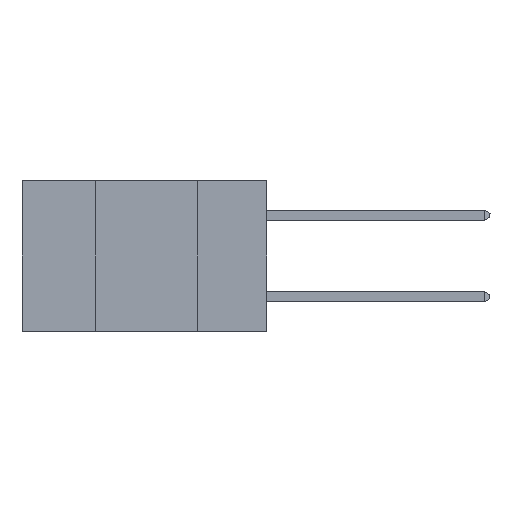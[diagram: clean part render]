
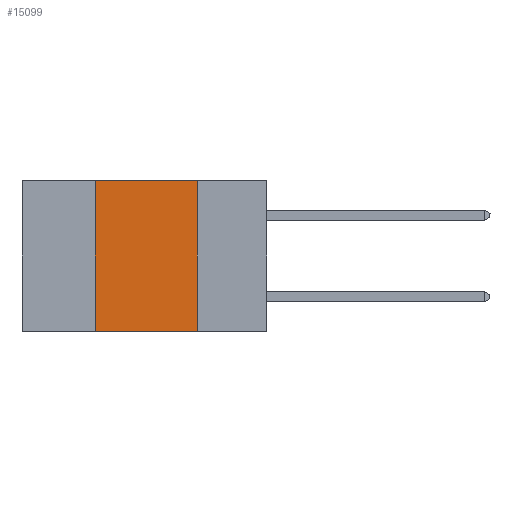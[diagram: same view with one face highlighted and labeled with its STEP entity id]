
A CAD part, left-side view. The second image highlights one B-rep face of the part: STEP entity #15099.
In plain terms, the highlighted planar face has unit normal (-1, 0, 0).
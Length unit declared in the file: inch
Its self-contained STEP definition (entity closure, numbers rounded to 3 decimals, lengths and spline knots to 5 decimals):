
#462 = CARTESIAN_POINT ( 'NONE',  ( 0., 0.42, 0. ) ) ;
#1358 = VECTOR ( 'NONE', #18595, 39.37008 ) ;
#1418 = EDGE_LOOP ( 'NONE', ( #22728, #8072, #20834, #23311 ) ) ;
#2671 = CARTESIAN_POINT ( 'NONE',  ( 0., 0.6, 0. ) ) ;
#7929 = VERTEX_POINT ( 'NONE', #19419 ) ;
#8072 = ORIENTED_EDGE ( 'NONE', *, *, #17607, .F. ) ;
#9355 = CARTESIAN_POINT ( 'NONE',  ( 0., 0.42, -0.37 ) ) ;
#9551 = VERTEX_POINT ( 'NONE', #22635 ) ;
#10447 = LINE ( 'NONE', #24664, #15486 ) ;
#10611 = DIRECTION ( 'NONE',  ( 0., 0., -1. ) ) ;
#10777 = LINE ( 'NONE', #20948, #1358 ) ;
#10842 = DIRECTION ( 'NONE',  ( 0., 0., 1. ) ) ;
#10975 = AXIS2_PLACEMENT_3D ( 'NONE', #2671, #24427, #10611 ) ;
#11197 = VERTEX_POINT ( 'NONE', #462 ) ;
#11290 = CARTESIAN_POINT ( 'NONE',  ( 0., 0.6, -0.37 ) ) ;
#11624 = VECTOR ( 'NONE', #19224, 39.37008 ) ;
#15099 = ADVANCED_FACE ( 'NONE', ( #20758 ), #20510, .F. ) ;
#15486 = VECTOR ( 'NONE', #10842, 39.37008 ) ;
#16877 = EDGE_CURVE ( 'NONE', #20349, #11197, #10447, .T. ) ;
#17493 = CARTESIAN_POINT ( 'NONE',  ( 0., 0.17, 0. ) ) ;
#17607 = EDGE_CURVE ( 'NONE', #11197, #7929, #10777, .T. ) ;
#18595 = DIRECTION ( 'NONE',  ( 0., -1., 0. ) ) ;
#19224 = DIRECTION ( 'NONE',  ( 0., -1., 0. ) ) ;
#19419 = CARTESIAN_POINT ( 'NONE',  ( 0., 0.17, 0. ) ) ;
#19437 = LINE ( 'NONE', #17493, #24631 ) ;
#20349 = VERTEX_POINT ( 'NONE', #9355 ) ;
#20510 = PLANE ( 'NONE',  #10975 ) ;
#20758 = FACE_OUTER_BOUND ( 'NONE', #1418, .T. ) ;
#20834 = ORIENTED_EDGE ( 'NONE', *, *, #16877, .F. ) ;
#20948 = CARTESIAN_POINT ( 'NONE',  ( 0., 0.6, 0. ) ) ;
#21173 = LINE ( 'NONE', #11290, #11624 ) ;
#21337 = EDGE_CURVE ( 'NONE', #7929, #9551, #19437, .T. ) ;
#22635 = CARTESIAN_POINT ( 'NONE',  ( 0., 0.17, -0.37 ) ) ;
#22728 = ORIENTED_EDGE ( 'NONE', *, *, #21337, .F. ) ;
#23311 = ORIENTED_EDGE ( 'NONE', *, *, #25178, .T. ) ;
#24427 = DIRECTION ( 'NONE',  ( 1., 0., 0. ) ) ;
#24631 = VECTOR ( 'NONE', #25446, 39.37008 ) ;
#24664 = CARTESIAN_POINT ( 'NONE',  ( 0., 0.42, 0. ) ) ;
#25178 = EDGE_CURVE ( 'NONE', #20349, #9551, #21173, .T. ) ;
#25446 = DIRECTION ( 'NONE',  ( 0., 0., -1. ) ) ;
